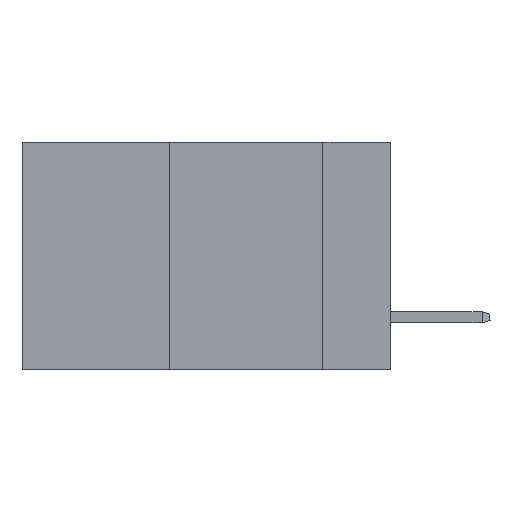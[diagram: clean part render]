
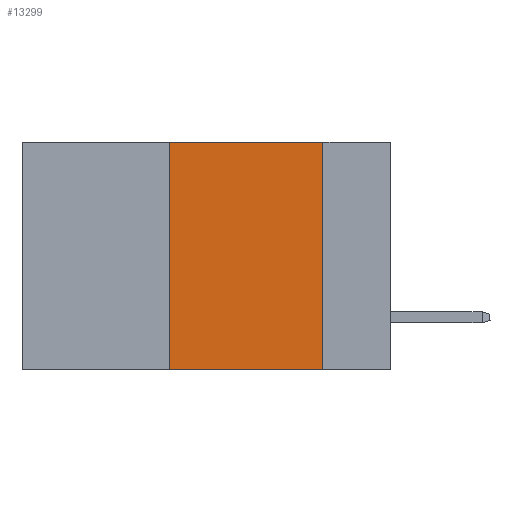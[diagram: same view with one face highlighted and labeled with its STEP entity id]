
A CAD part, left-side view. The second image highlights one B-rep face of the part: STEP entity #13299.
In plain terms, the highlighted planar face has unit normal (-1, 0, 0).
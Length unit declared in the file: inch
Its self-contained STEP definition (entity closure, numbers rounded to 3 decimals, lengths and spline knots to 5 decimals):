
#45 = VECTOR ( 'NONE', #11681, 39.37008 ) ;
#57 = DIRECTION ( 'NONE',  ( 0., -1., 0. ) ) ;
#644 = PLANE ( 'NONE',  #5086 ) ;
#692 = DIRECTION ( 'NONE',  ( 0., 0., 1. ) ) ;
#1071 = DIRECTION ( 'NONE',  ( 0., -1., 0. ) ) ;
#1751 = CARTESIAN_POINT ( 'NONE',  ( 0., 0.11, 0. ) ) ;
#2084 = VECTOR ( 'NONE', #57, 39.37008 ) ;
#2147 = ORIENTED_EDGE ( 'NONE', *, *, #13369, .F. ) ;
#2279 = DIRECTION ( 'NONE',  ( 0., 0., -1. ) ) ;
#2695 = EDGE_CURVE ( 'NONE', #10701, #4415, #17478, .T. ) ;
#2998 = LINE ( 'NONE', #7343, #2084 ) ;
#3800 = EDGE_CURVE ( 'NONE', #10701, #4830, #2998, .T. ) ;
#3810 = VECTOR ( 'NONE', #692, 39.37008 ) ;
#4085 = EDGE_CURVE ( 'NONE', #15249, #4830, #10509, .T. ) ;
#4415 = VERTEX_POINT ( 'NONE', #15660 ) ;
#4830 = VERTEX_POINT ( 'NONE', #18692 ) ;
#4971 = CARTESIAN_POINT ( 'NONE',  ( 0., 0.36, 0. ) ) ;
#5086 = AXIS2_PLACEMENT_3D ( 'NONE', #9421, #11019, #2279 ) ;
#5184 = EDGE_LOOP ( 'NONE', ( #16367, #2147, #16814, #8953 ) ) ;
#5825 = CARTESIAN_POINT ( 'NONE',  ( 0., 0.36, -0.37 ) ) ;
#6328 = LINE ( 'NONE', #9794, #7483 ) ;
#7343 = CARTESIAN_POINT ( 'NONE',  ( 0., 0.6, -0.37 ) ) ;
#7483 = VECTOR ( 'NONE', #1071, 39.37008 ) ;
#8712 = CARTESIAN_POINT ( 'NONE',  ( 0., 0.11, 0. ) ) ;
#8953 = ORIENTED_EDGE ( 'NONE', *, *, #3800, .T. ) ;
#9421 = CARTESIAN_POINT ( 'NONE',  ( 0., 0.6, 0. ) ) ;
#9794 = CARTESIAN_POINT ( 'NONE',  ( 0., 0.6, 0. ) ) ;
#10509 = LINE ( 'NONE', #8712, #45 ) ;
#10701 = VERTEX_POINT ( 'NONE', #5825 ) ;
#11019 = DIRECTION ( 'NONE',  ( 1., 0., 0. ) ) ;
#11377 = FACE_OUTER_BOUND ( 'NONE', #5184, .T. ) ;
#11681 = DIRECTION ( 'NONE',  ( 0., 0., -1. ) ) ;
#13299 = ADVANCED_FACE ( 'NONE', ( #11377 ), #644, .F. ) ;
#13369 = EDGE_CURVE ( 'NONE', #4415, #15249, #6328, .T. ) ;
#15249 = VERTEX_POINT ( 'NONE', #1751 ) ;
#15660 = CARTESIAN_POINT ( 'NONE',  ( 0., 0.36, 0. ) ) ;
#16367 = ORIENTED_EDGE ( 'NONE', *, *, #4085, .F. ) ;
#16814 = ORIENTED_EDGE ( 'NONE', *, *, #2695, .F. ) ;
#17478 = LINE ( 'NONE', #4971, #3810 ) ;
#18692 = CARTESIAN_POINT ( 'NONE',  ( 0., 0.11, -0.37 ) ) ;
